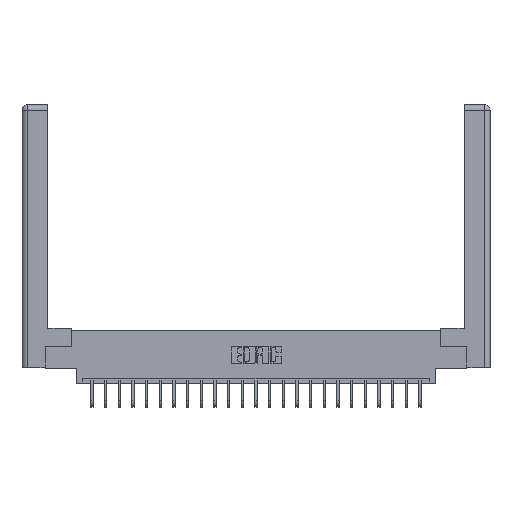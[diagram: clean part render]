
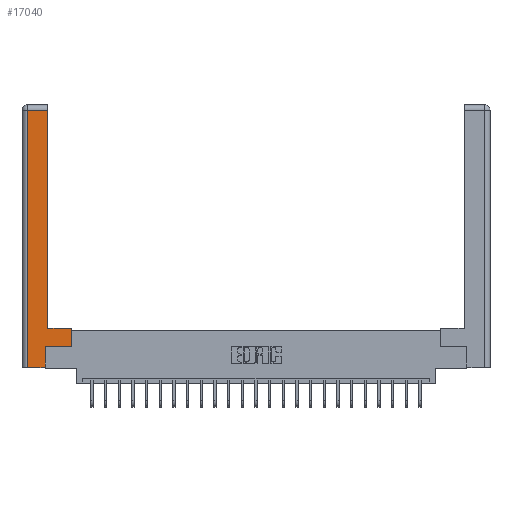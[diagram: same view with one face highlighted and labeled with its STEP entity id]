
A CAD part, top view. The second image highlights one B-rep face of the part: STEP entity #17040.
In plain terms, the highlighted planar face has unit normal (0, 0, 1).
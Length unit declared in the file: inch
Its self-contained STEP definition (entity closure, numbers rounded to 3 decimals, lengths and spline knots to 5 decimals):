
#74 = DIRECTION ( 'NONE',  ( -1., 0., 0. ) ) ;
#486 = LINE ( 'NONE', #23975, #3916 ) ;
#673 = VECTOR ( 'NONE', #19969, 39.37008 ) ;
#891 = VECTOR ( 'NONE', #7967, 39.37008 ) ;
#1048 = CARTESIAN_POINT ( 'NONE',  ( 0.565, 0.45, 0. ) ) ;
#1103 = ORIENTED_EDGE ( 'NONE', *, *, #20711, .T. ) ;
#1279 = ORIENTED_EDGE ( 'NONE', *, *, #14429, .T. ) ;
#2367 = VERTEX_POINT ( 'NONE', #10175 ) ;
#2459 = ORIENTED_EDGE ( 'NONE', *, *, #11779, .T. ) ;
#2487 = ORIENTED_EDGE ( 'NONE', *, *, #16266, .T. ) ;
#2581 = VERTEX_POINT ( 'NONE', #20758 ) ;
#3114 = CARTESIAN_POINT ( 'NONE',  ( 0.295, 0.45, 0. ) ) ;
#3213 = VERTEX_POINT ( 'NONE', #16973 ) ;
#3916 = VECTOR ( 'NONE', #17692, 39.37008 ) ;
#4467 = LINE ( 'NONE', #24116, #673 ) ;
#4648 = EDGE_CURVE ( 'NONE', #11011, #2367, #22143, .T. ) ;
#4990 = CARTESIAN_POINT ( 'NONE',  ( 0.265, 0., 0. ) ) ;
#5857 = ORIENTED_EDGE ( 'NONE', *, *, #24248, .T. ) ;
#7445 = VERTEX_POINT ( 'NONE', #22992 ) ;
#7967 = DIRECTION ( 'NONE',  ( 0., 1., 0. ) ) ;
#7992 = DIRECTION ( 'NONE',  ( 1., 0., 0. ) ) ;
#8025 = CARTESIAN_POINT ( 'NONE',  ( 0.265, 0., 0. ) ) ;
#8090 = DIRECTION ( 'NONE',  ( 0., 0., -1. ) ) ;
#8226 = LINE ( 'NONE', #8025, #18364 ) ;
#9452 = DIRECTION ( 'NONE',  ( 0., 1., 0. ) ) ;
#9595 = VECTOR ( 'NONE', #12404, 39.37008 ) ;
#9677 = VERTEX_POINT ( 'NONE', #4990 ) ;
#10118 = DIRECTION ( 'NONE',  ( 0., 1., 0. ) ) ;
#10175 = CARTESIAN_POINT ( 'NONE',  ( 0.295, 2.94, 0. ) ) ;
#10235 = LINE ( 'NONE', #10352, #9595 ) ;
#10352 = CARTESIAN_POINT ( 'NONE',  ( 0.295, 0.45, 0. ) ) ;
#11011 = VERTEX_POINT ( 'NONE', #3114 ) ;
#11363 = VECTOR ( 'NONE', #9452, 39.37008 ) ;
#11635 = CARTESIAN_POINT ( 'NONE',  ( 0.0615, 2.94, 0. ) ) ;
#11779 = EDGE_CURVE ( 'NONE', #25879, #3213, #20478, .T. ) ;
#12051 = CARTESIAN_POINT ( 'NONE',  ( 0., 0., 0. ) ) ;
#12088 = CARTESIAN_POINT ( 'NONE',  ( 0.265, 0.245, 0. ) ) ;
#12404 = DIRECTION ( 'NONE',  ( -1., 0., 0. ) ) ;
#12774 = EDGE_LOOP ( 'NONE', ( #16198, #5857, #25151, #2487, #1279, #1103, #2459, #15658 ) ) ;
#13250 = EDGE_CURVE ( 'NONE', #3213, #11011, #10235, .T. ) ;
#13659 = EDGE_CURVE ( 'NONE', #14269, #7445, #486, .T. ) ;
#13971 = LINE ( 'NONE', #12088, #22518 ) ;
#14004 = CARTESIAN_POINT ( 'NONE',  ( 0.565, 0.245, 0. ) ) ;
#14269 = VERTEX_POINT ( 'NONE', #11635 ) ;
#14429 = EDGE_CURVE ( 'NONE', #9677, #2581, #13971, .T. ) ;
#14573 = AXIS2_PLACEMENT_3D ( 'NONE', #12051, #8090, #74 ) ;
#15658 = ORIENTED_EDGE ( 'NONE', *, *, #13250, .T. ) ;
#15744 = LINE ( 'NONE', #14004, #16697 ) ;
#16198 = ORIENTED_EDGE ( 'NONE', *, *, #4648, .T. ) ;
#16266 = EDGE_CURVE ( 'NONE', #7445, #9677, #8226, .T. ) ;
#16697 = VECTOR ( 'NONE', #7992, 39.37008 ) ;
#16973 = CARTESIAN_POINT ( 'NONE',  ( 0.565, 0.45, 0. ) ) ;
#17040 = ADVANCED_FACE ( 'NONE', ( #22899 ), #24190, .F. ) ;
#17692 = DIRECTION ( 'NONE',  ( 0., -1., 0. ) ) ;
#18107 = DIRECTION ( 'NONE',  ( 1., 0., 0. ) ) ;
#18364 = VECTOR ( 'NONE', #18107, 39.37008 ) ;
#19969 = DIRECTION ( 'NONE',  ( -1., 0., 0. ) ) ;
#20478 = LINE ( 'NONE', #1048, #891 ) ;
#20711 = EDGE_CURVE ( 'NONE', #2581, #25879, #15744, .T. ) ;
#20758 = CARTESIAN_POINT ( 'NONE',  ( 0.265, 0.245, 0. ) ) ;
#21454 = CARTESIAN_POINT ( 'NONE',  ( 0.295, 3., 0. ) ) ;
#22143 = LINE ( 'NONE', #21454, #11363 ) ;
#22518 = VECTOR ( 'NONE', #10118, 39.37008 ) ;
#22816 = CARTESIAN_POINT ( 'NONE',  ( 0.565, 0.245, 0. ) ) ;
#22899 = FACE_OUTER_BOUND ( 'NONE', #12774, .T. ) ;
#22992 = CARTESIAN_POINT ( 'NONE',  ( 0.0615, 0., 0. ) ) ;
#23975 = CARTESIAN_POINT ( 'NONE',  ( 0.0615, 0., 0. ) ) ;
#24116 = CARTESIAN_POINT ( 'NONE',  ( 0.0615, 2.94, 0. ) ) ;
#24190 = PLANE ( 'NONE',  #14573 ) ;
#24248 = EDGE_CURVE ( 'NONE', #2367, #14269, #4467, .T. ) ;
#25151 = ORIENTED_EDGE ( 'NONE', *, *, #13659, .T. ) ;
#25879 = VERTEX_POINT ( 'NONE', #22816 ) ;
